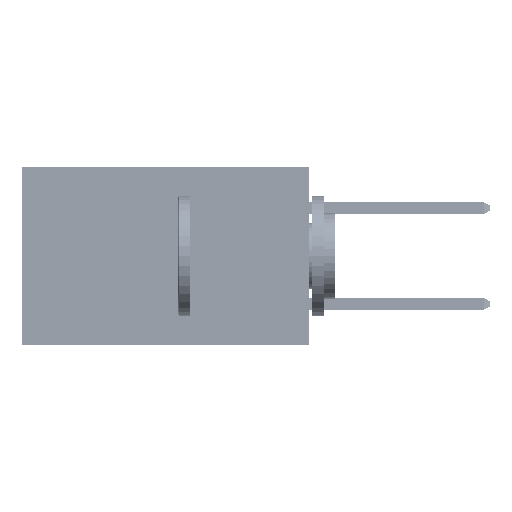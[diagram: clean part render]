
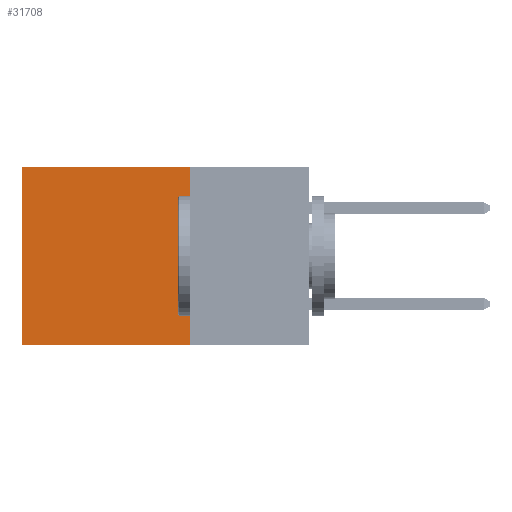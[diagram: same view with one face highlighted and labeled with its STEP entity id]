
A CAD part, left-side view. The second image highlights one B-rep face of the part: STEP entity #31708.
In plain terms, the highlighted planar face has unit normal (-1, 0, 0).
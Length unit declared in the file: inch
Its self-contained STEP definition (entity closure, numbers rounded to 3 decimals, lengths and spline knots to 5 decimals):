
#1761 = ORIENTED_EDGE ( 'NONE', *, *, #7732, .F. ) ;
#2291 = CARTESIAN_POINT ( 'NONE',  ( 0.2875, 0.25, 0. ) ) ;
#3428 = DIRECTION ( 'NONE',  ( 1., 0., 0. ) ) ;
#5084 = VERTEX_POINT ( 'NONE', #26234 ) ;
#7732 = EDGE_CURVE ( 'NONE', #45318, #21322, #25511, .T. ) ;
#8992 = VECTOR ( 'NONE', #32886, 39.37008 ) ;
#10210 = VECTOR ( 'NONE', #22827, 39.37008 ) ;
#10505 = DIRECTION ( 'NONE',  ( 0., 0., -1. ) ) ;
#11607 = PLANE ( 'NONE',  #22945 ) ;
#11947 = CARTESIAN_POINT ( 'NONE',  ( 0.2875, 0.25, -0.37 ) ) ;
#13676 = FACE_OUTER_BOUND ( 'NONE', #14887, .T. ) ;
#14542 = VERTEX_POINT ( 'NONE', #35723 ) ;
#14887 = EDGE_LOOP ( 'NONE', ( #34052, #43649, #1761, #29798 ) ) ;
#18479 = EDGE_CURVE ( 'NONE', #45318, #14542, #47801, .T. ) ;
#18698 = CARTESIAN_POINT ( 'NONE',  ( 0.2875, 0.25, 0. ) ) ;
#19216 = EDGE_CURVE ( 'NONE', #21322, #5084, #28991, .T. ) ;
#21322 = VERTEX_POINT ( 'NONE', #11947 ) ;
#22827 = DIRECTION ( 'NONE',  ( 0., 1., 0. ) ) ;
#22945 = AXIS2_PLACEMENT_3D ( 'NONE', #18698, #3428, #30165 ) ;
#25502 = CARTESIAN_POINT ( 'NONE',  ( 0.2875, 0.25, -0.37 ) ) ;
#25511 = LINE ( 'NONE', #39952, #26678 ) ;
#26234 = CARTESIAN_POINT ( 'NONE',  ( 0.2875, 0.6, -0.37 ) ) ;
#26678 = VECTOR ( 'NONE', #10505, 39.37008 ) ;
#28991 = LINE ( 'NONE', #25502, #8992 ) ;
#29798 = ORIENTED_EDGE ( 'NONE', *, *, #18479, .T. ) ;
#30165 = DIRECTION ( 'NONE',  ( 0., 0., -1. ) ) ;
#31708 = ADVANCED_FACE ( 'NONE', ( #13676 ), #11607, .F. ) ;
#31721 = CARTESIAN_POINT ( 'NONE',  ( 0.2875, 0.6, 0. ) ) ;
#32737 = EDGE_CURVE ( 'NONE', #14542, #5084, #37709, .T. ) ;
#32886 = DIRECTION ( 'NONE',  ( 0., 1., 0. ) ) ;
#34052 = ORIENTED_EDGE ( 'NONE', *, *, #32737, .T. ) ;
#35529 = DIRECTION ( 'NONE',  ( 0., 0., -1. ) ) ;
#35723 = CARTESIAN_POINT ( 'NONE',  ( 0.2875, 0.6, 0. ) ) ;
#37709 = LINE ( 'NONE', #31721, #42978 ) ;
#39952 = CARTESIAN_POINT ( 'NONE',  ( 0.2875, 0.25, 0. ) ) ;
#42978 = VECTOR ( 'NONE', #35529, 39.37008 ) ;
#43649 = ORIENTED_EDGE ( 'NONE', *, *, #19216, .F. ) ;
#45030 = CARTESIAN_POINT ( 'NONE',  ( 0.2875, 0.25, 0. ) ) ;
#45318 = VERTEX_POINT ( 'NONE', #2291 ) ;
#47801 = LINE ( 'NONE', #45030, #10210 ) ;
